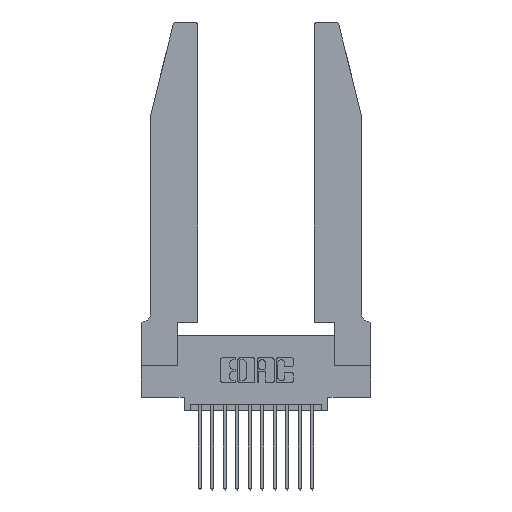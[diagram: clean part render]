
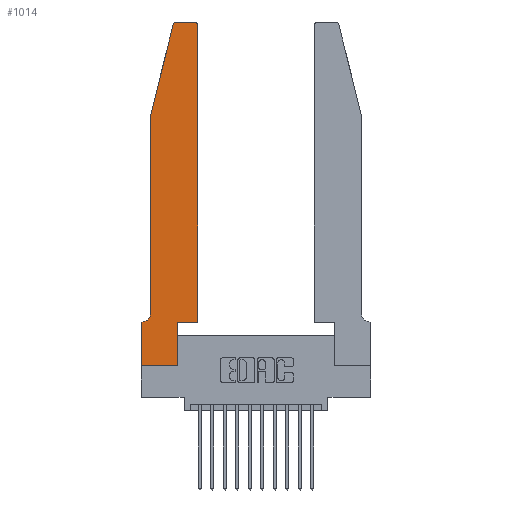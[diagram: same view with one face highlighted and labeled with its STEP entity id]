
A CAD part, top view. The second image highlights one B-rep face of the part: STEP entity #1014.
In plain terms, the highlighted planar face has unit normal (0, 0, 1).
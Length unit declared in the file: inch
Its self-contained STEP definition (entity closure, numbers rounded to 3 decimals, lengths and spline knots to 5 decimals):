
#158 = DIRECTION ( 'NONE',  ( -1., 0., 0. ) ) ;
#179 = EDGE_CURVE ( 'NONE', #6791, #7920, #11487, .T. ) ;
#214 = VERTEX_POINT ( 'NONE', #4368 ) ;
#378 = DIRECTION ( 'NONE',  ( 1., 0., 0. ) ) ;
#592 = DIRECTION ( 'NONE',  ( 1., 0., 0. ) ) ;
#764 = VECTOR ( 'NONE', #7283, 39.37008 ) ;
#919 = VECTOR ( 'NONE', #2979, 39.37008 ) ;
#985 = VERTEX_POINT ( 'NONE', #4479 ) ;
#1014 = ADVANCED_FACE ( 'NONE', ( #10072 ), #14950, .T. ) ;
#1256 = VECTOR ( 'NONE', #12941, 39.37008 ) ;
#1391 = LINE ( 'NONE', #7148, #14589 ) ;
#1452 = DIRECTION ( 'NONE',  ( 0., -1., 0. ) ) ;
#1624 = EDGE_CURVE ( 'NONE', #15207, #12956, #12633, .T. ) ;
#1742 = EDGE_CURVE ( 'NONE', #15067, #2129, #14746, .T. ) ;
#1833 = LINE ( 'NONE', #12092, #12048 ) ;
#2095 = CARTESIAN_POINT ( 'NONE',  ( 0., 0., 0.37 ) ) ;
#2129 = VERTEX_POINT ( 'NONE', #4649 ) ;
#2458 = VERTEX_POINT ( 'NONE', #15553 ) ;
#2979 = DIRECTION ( 'NONE',  ( -1., 0., 0. ) ) ;
#3116 = ORIENTED_EDGE ( 'NONE', *, *, #14956, .T. ) ;
#3417 = ORIENTED_EDGE ( 'NONE', *, *, #3657, .T. ) ;
#3496 = CARTESIAN_POINT ( 'NONE',  ( 0.4505, 0.35, 0.37 ) ) ;
#3519 = ORIENTED_EDGE ( 'NONE', *, *, #9487, .T. ) ;
#3570 = AXIS2_PLACEMENT_3D ( 'NONE', #14238, #6542, #15481 ) ;
#3617 = AXIS2_PLACEMENT_3D ( 'NONE', #16007, #8449, #158 ) ;
#3657 = EDGE_CURVE ( 'NONE', #16363, #8711, #10296, .T. ) ;
#3658 = ORIENTED_EDGE ( 'NONE', *, *, #14919, .T. ) ;
#3724 = ORIENTED_EDGE ( 'NONE', *, *, #8786, .T. ) ;
#3775 = ORIENTED_EDGE ( 'NONE', *, *, #1742, .T. ) ;
#3814 = ORIENTED_EDGE ( 'NONE', *, *, #13886, .T. ) ;
#3883 = ORIENTED_EDGE ( 'NONE', *, *, #1624, .T. ) ;
#3914 = ORIENTED_EDGE ( 'NONE', *, *, #15462, .T. ) ;
#4002 = ORIENTED_EDGE ( 'NONE', *, *, #179, .T. ) ;
#4155 = CARTESIAN_POINT ( 'NONE',  ( 0.4505, 2.72, 0.37 ) ) ;
#4368 = CARTESIAN_POINT ( 'NONE',  ( 0.4205, 2.75, 0.37 ) ) ;
#4479 = CARTESIAN_POINT ( 'NONE',  ( 0.0755, 2., 0.37 ) ) ;
#4553 = CARTESIAN_POINT ( 'NONE',  ( 0.0755, 2., 0.37 ) ) ;
#4558 = LINE ( 'NONE', #4553, #764 ) ;
#4649 = CARTESIAN_POINT ( 'NONE',  ( 0., 0.35, 0.37 ) ) ;
#5170 = ORIENTED_EDGE ( 'NONE', *, *, #8482, .T. ) ;
#5613 = CARTESIAN_POINT ( 'NONE',  ( 0.25487, 2.72718, 0.37 ) ) ;
#5720 = VECTOR ( 'NONE', #378, 39.37008 ) ;
#6236 = VECTOR ( 'NONE', #13897, 39.37008 ) ;
#6542 = DIRECTION ( 'NONE',  ( 0., 0., 1. ) ) ;
#6585 = CARTESIAN_POINT ( 'NONE',  ( 0.2865, 0.35, 0.37 ) ) ;
#6742 = CARTESIAN_POINT ( 'NONE',  ( 0.4205, 2.72, 0.37 ) ) ;
#6791 = VERTEX_POINT ( 'NONE', #6585 ) ;
#7092 = DIRECTION ( 'NONE',  ( 0., 0., 1. ) ) ;
#7111 = CARTESIAN_POINT ( 'NONE',  ( 0., 0.35, 0.37 ) ) ;
#7148 = CARTESIAN_POINT ( 'NONE',  ( 0., 0., 0.37 ) ) ;
#7283 = DIRECTION ( 'NONE',  ( -0.239, -0.971, 0. ) ) ;
#7294 = CARTESIAN_POINT ( 'NONE',  ( 0.0055, 0.35, 0.37 ) ) ;
#7360 = CARTESIAN_POINT ( 'NONE',  ( 0.4505, 0.35, 0.37 ) ) ;
#7920 = VERTEX_POINT ( 'NONE', #15595 ) ;
#8044 = DIRECTION ( 'NONE',  ( 1., 0., 0. ) ) ;
#8072 = DIRECTION ( 'NONE',  ( 1., 0., 0. ) ) ;
#8449 = DIRECTION ( 'NONE',  ( 0., 0., -1. ) ) ;
#8471 = DIRECTION ( 'NONE',  ( -1., 0., 0. ) ) ;
#8482 = EDGE_CURVE ( 'NONE', #12956, #6791, #8958, .T. ) ;
#8711 = VERTEX_POINT ( 'NONE', #5613 ) ;
#8786 = EDGE_CURVE ( 'NONE', #2458, #15067, #14660, .T. ) ;
#8870 = EDGE_CURVE ( 'NONE', #7920, #14327, #16402, .T. ) ;
#8958 = LINE ( 'NONE', #11677, #1256 ) ;
#9487 = EDGE_CURVE ( 'NONE', #8711, #985, #4558, .T. ) ;
#9611 = CARTESIAN_POINT ( 'NONE',  ( 0.0755, 0.35, 0.37 ) ) ;
#10054 = CARTESIAN_POINT ( 'NONE',  ( 0.2865, 0., 0.37 ) ) ;
#10072 = FACE_OUTER_BOUND ( 'NONE', #10898, .T. ) ;
#10147 = CARTESIAN_POINT ( 'NONE',  ( 0., 0., 0.37 ) ) ;
#10296 = CIRCLE ( 'NONE', #3570, 0.03 ) ;
#10682 = VECTOR ( 'NONE', #8044, 39.37008 ) ;
#10898 = EDGE_LOOP ( 'NONE', ( #3116, #3417, #3519, #3658, #3724, #3775, #3814, #3883, #5170, #4002, #14923, #3914 ) ) ;
#11449 = VECTOR ( 'NONE', #8471, 39.37008 ) ;
#11487 = LINE ( 'NONE', #7360, #10682 ) ;
#11665 = LINE ( 'NONE', #13456, #919 ) ;
#11677 = CARTESIAN_POINT ( 'NONE',  ( 0.2865, 0.35, 0.37 ) ) ;
#12048 = VECTOR ( 'NONE', #1452, 39.37008 ) ;
#12092 = CARTESIAN_POINT ( 'NONE',  ( 0.0755, 2., 0.37 ) ) ;
#12633 = LINE ( 'NONE', #10147, #5720 ) ;
#12941 = DIRECTION ( 'NONE',  ( 0., 1., 0. ) ) ;
#12956 = VERTEX_POINT ( 'NONE', #10054 ) ;
#13257 = AXIS2_PLACEMENT_3D ( 'NONE', #6742, #15665, #8072 ) ;
#13456 = CARTESIAN_POINT ( 'NONE',  ( 0.2605, 2.75, 0.37 ) ) ;
#13801 = CIRCLE ( 'NONE', #13257, 0.03 ) ;
#13886 = EDGE_CURVE ( 'NONE', #2129, #15207, #1391, .T. ) ;
#13897 = DIRECTION ( 'NONE',  ( 0., 1., 0. ) ) ;
#14238 = CARTESIAN_POINT ( 'NONE',  ( 0.284, 2.72, 0.37 ) ) ;
#14327 = VERTEX_POINT ( 'NONE', #4155 ) ;
#14589 = VECTOR ( 'NONE', #14785, 39.37008 ) ;
#14660 = CIRCLE ( 'NONE', #3617, 0.07 ) ;
#14746 = LINE ( 'NONE', #9611, #11449 ) ;
#14785 = DIRECTION ( 'NONE',  ( 0., -1., 0. ) ) ;
#14919 = EDGE_CURVE ( 'NONE', #985, #2458, #1833, .T. ) ;
#14923 = ORIENTED_EDGE ( 'NONE', *, *, #8870, .T. ) ;
#14950 = PLANE ( 'NONE',  #17059 ) ;
#14956 = EDGE_CURVE ( 'NONE', #214, #16363, #11665, .T. ) ;
#15067 = VERTEX_POINT ( 'NONE', #7294 ) ;
#15207 = VERTEX_POINT ( 'NONE', #2095 ) ;
#15462 = EDGE_CURVE ( 'NONE', #14327, #214, #13801, .T. ) ;
#15481 = DIRECTION ( 'NONE',  ( 1., 0., 0. ) ) ;
#15553 = CARTESIAN_POINT ( 'NONE',  ( 0.0755, 0.42, 0.37 ) ) ;
#15595 = CARTESIAN_POINT ( 'NONE',  ( 0.4505, 0.35, 0.37 ) ) ;
#15665 = DIRECTION ( 'NONE',  ( 0., 0., 1. ) ) ;
#16007 = CARTESIAN_POINT ( 'NONE',  ( 0.0055, 0.42, 0.37 ) ) ;
#16363 = VERTEX_POINT ( 'NONE', #16801 ) ;
#16402 = LINE ( 'NONE', #3496, #6236 ) ;
#16801 = CARTESIAN_POINT ( 'NONE',  ( 0.284, 2.75, 0.37 ) ) ;
#17059 = AXIS2_PLACEMENT_3D ( 'NONE', #7111, #7092, #592 ) ;
